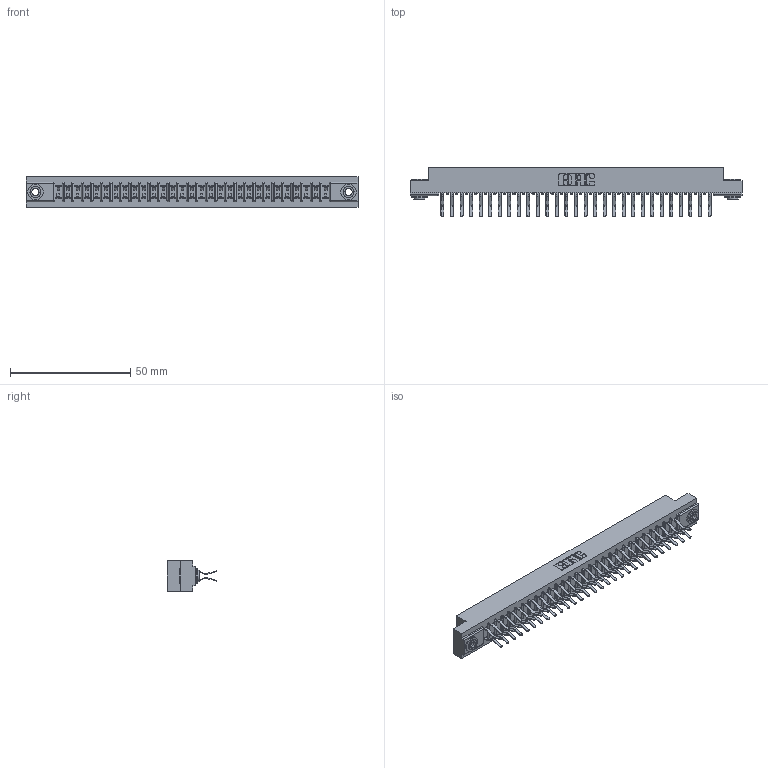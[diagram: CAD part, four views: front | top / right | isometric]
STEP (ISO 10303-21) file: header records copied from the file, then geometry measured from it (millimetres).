
FILE_DESCRIPTION (( 'STEP AP203' ), '1' );
FILE_NAME ('307-058-560-203.STEP', '2019-09-06T14:41:14', ( '' ), ( '' ), 'SwSTEP 2.0', 'SolidWorks 2016', '' );
FILE_SCHEMA (( 'CONFIG_CONTROL_DESIGN' ));
Length unit declared in the file: inch
Products named in the file (4): 307-290-001_560; 307 Part_.156 Dia Mounting Holes; 345-250-002_345-250-002-102; 307-058-560-203
Assembly tree (61 placements, depth 2):
  307-058-560-203
    307 Part_.156 Dia Mounting Holes
    307-290-001_560  x58
    345-250-002_345-250-002-102  x2
Bounding box: 137.92 x 20.73 x 12.7 mm (x, y, z)
Volume: 14647.8 mm3; surface area: 18299.8 mm2
Topology: 61 solids, 61 shells, 3100 faces, 8671 edges, 5618 vertices
Faces by surface type: plane 2008, cylinder 1024, sphere 60, cone 8
Entity records: 28561 total; most frequent: CARTESIAN_POINT 4658, ORIENTED_EDGE 4606, DIRECTION 4583, EDGE_CURVE 2303, LINE 1753, VECTOR 1753, VERTEX_POINT 1490, AXIS2_PLACEMENT_3D 1415
